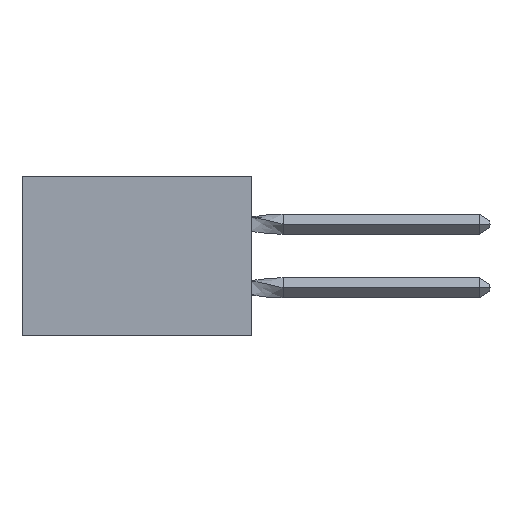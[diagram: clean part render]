
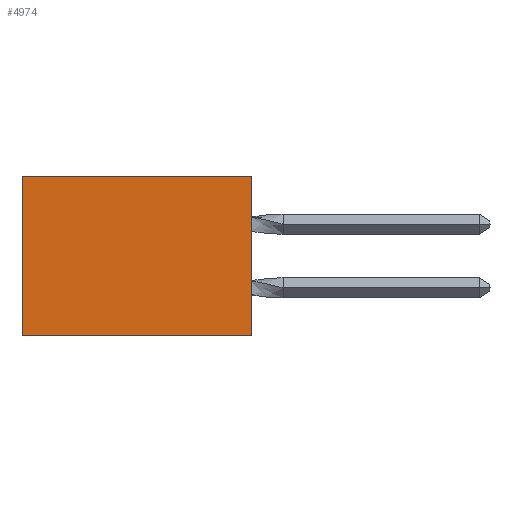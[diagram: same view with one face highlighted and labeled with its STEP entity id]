
A CAD part, left-side view. The second image highlights one B-rep face of the part: STEP entity #4974.
In plain terms, the highlighted planar face has unit normal (-1, 0, 0).
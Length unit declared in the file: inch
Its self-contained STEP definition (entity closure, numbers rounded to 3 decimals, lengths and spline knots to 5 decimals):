
#1394 = DIRECTION ( 'NONE',  ( 0., 0., -1. ) ) ;
#2819 = CARTESIAN_POINT ( 'NONE',  ( 0.305, 0., -0.5 ) ) ;
#2866 = VERTEX_POINT ( 'NONE', #14750 ) ;
#2892 = LINE ( 'NONE', #21457, #22884 ) ;
#4407 = VERTEX_POINT ( 'NONE', #17975 ) ;
#4974 = ADVANCED_FACE ( 'NONE', ( #22308 ), #7693, .F. ) ;
#5387 = VERTEX_POINT ( 'NONE', #20628 ) ;
#5645 = CARTESIAN_POINT ( 'NONE',  ( 0.305, 0.72, -0.5 ) ) ;
#5790 = LINE ( 'NONE', #2819, #22225 ) ;
#5867 = LINE ( 'NONE', #9998, #20042 ) ;
#6694 = EDGE_CURVE ( 'NONE', #4407, #2866, #2892, .T. ) ;
#7555 = AXIS2_PLACEMENT_3D ( 'NONE', #13581, #13840, #1394 ) ;
#7693 = PLANE ( 'NONE',  #7555 ) ;
#9998 = CARTESIAN_POINT ( 'NONE',  ( 0.305, 0., -0.5 ) ) ;
#10952 = VECTOR ( 'NONE', #24020, 39.37008 ) ;
#11293 = ORIENTED_EDGE ( 'NONE', *, *, #23505, .T. ) ;
#12262 = CARTESIAN_POINT ( 'NONE',  ( 0.305, 0., -0.5 ) ) ;
#13581 = CARTESIAN_POINT ( 'NONE',  ( 0.305, 0., -0.5 ) ) ;
#13840 = DIRECTION ( 'NONE',  ( 1., 0., 0. ) ) ;
#13905 = VERTEX_POINT ( 'NONE', #12262 ) ;
#14750 = CARTESIAN_POINT ( 'NONE',  ( 0.305, 0.72, 0. ) ) ;
#15334 = DIRECTION ( 'NONE',  ( 0., 1., 0. ) ) ;
#15570 = ORIENTED_EDGE ( 'NONE', *, *, #6694, .T. ) ;
#16199 = DIRECTION ( 'NONE',  ( 0., 1., 0. ) ) ;
#16412 = LINE ( 'NONE', #5645, #10952 ) ;
#16566 = EDGE_CURVE ( 'NONE', #13905, #5387, #5867, .T. ) ;
#16662 = EDGE_LOOP ( 'NONE', ( #11293, #21696, #17002, #15570 ) ) ;
#17002 = ORIENTED_EDGE ( 'NONE', *, *, #22610, .F. ) ;
#17975 = CARTESIAN_POINT ( 'NONE',  ( 0.305, 0., 0. ) ) ;
#19288 = DIRECTION ( 'NONE',  ( 0., 0., -1. ) ) ;
#20042 = VECTOR ( 'NONE', #16199, 39.37008 ) ;
#20628 = CARTESIAN_POINT ( 'NONE',  ( 0.305, 0.72, -0.5 ) ) ;
#21457 = CARTESIAN_POINT ( 'NONE',  ( 0.305, 0., 0. ) ) ;
#21696 = ORIENTED_EDGE ( 'NONE', *, *, #16566, .F. ) ;
#22225 = VECTOR ( 'NONE', #19288, 39.37008 ) ;
#22308 = FACE_OUTER_BOUND ( 'NONE', #16662, .T. ) ;
#22610 = EDGE_CURVE ( 'NONE', #4407, #13905, #5790, .T. ) ;
#22884 = VECTOR ( 'NONE', #15334, 39.37008 ) ;
#23505 = EDGE_CURVE ( 'NONE', #2866, #5387, #16412, .T. ) ;
#24020 = DIRECTION ( 'NONE',  ( 0., 0., -1. ) ) ;
